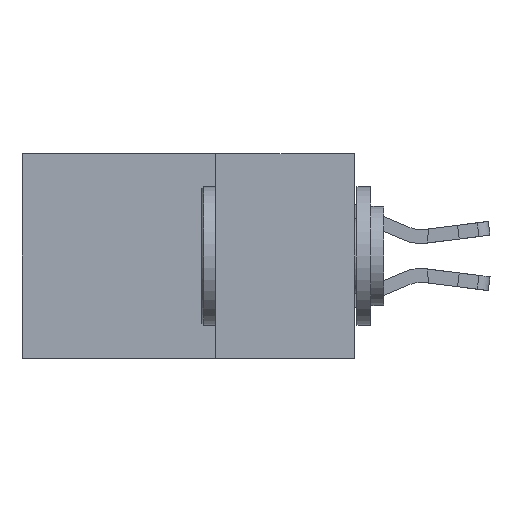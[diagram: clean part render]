
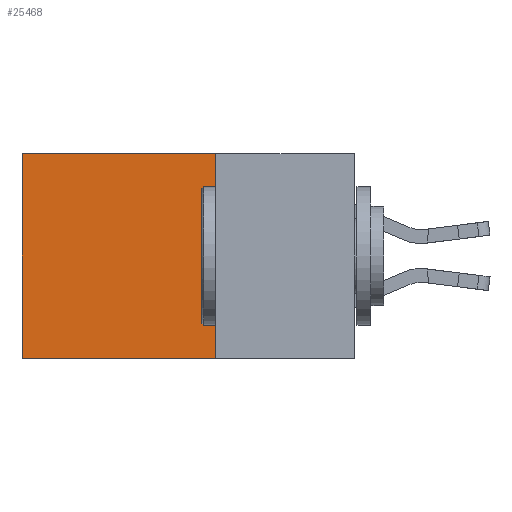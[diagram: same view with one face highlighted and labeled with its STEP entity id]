
A CAD part, left-side view. The second image highlights one B-rep face of the part: STEP entity #25468.
In plain terms, the highlighted planar face has unit normal (-1, 0, 0).
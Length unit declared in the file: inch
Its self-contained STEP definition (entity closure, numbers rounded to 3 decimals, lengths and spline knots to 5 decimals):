
#117 = CARTESIAN_POINT ( 'NONE',  ( 0.298, 0.25, 0. ) ) ;
#673 = EDGE_LOOP ( 'NONE', ( #4429, #25153, #6160, #6179 ) ) ;
#1301 = DIRECTION ( 'NONE',  ( 0., 0., -1. ) ) ;
#4429 = ORIENTED_EDGE ( 'NONE', *, *, #16541, .T. ) ;
#4519 = CARTESIAN_POINT ( 'NONE',  ( 0.298, 0.25, -0.37 ) ) ;
#5202 = LINE ( 'NONE', #8693, #21627 ) ;
#5887 = CARTESIAN_POINT ( 'NONE',  ( 0.298, 0.6, 0. ) ) ;
#6160 = ORIENTED_EDGE ( 'NONE', *, *, #19149, .F. ) ;
#6179 = ORIENTED_EDGE ( 'NONE', *, *, #23995, .T. ) ;
#6686 = VERTEX_POINT ( 'NONE', #5887 ) ;
#8188 = CARTESIAN_POINT ( 'NONE',  ( 0.298, 0.6, 0. ) ) ;
#8596 = FACE_OUTER_BOUND ( 'NONE', #673, .T. ) ;
#8693 = CARTESIAN_POINT ( 'NONE',  ( 0.298, 0.25, 0. ) ) ;
#9989 = CARTESIAN_POINT ( 'NONE',  ( 0.298, 0.25, 0. ) ) ;
#12301 = LINE ( 'NONE', #8188, #12620 ) ;
#12393 = DIRECTION ( 'NONE',  ( 1., 0., 0. ) ) ;
#12620 = VECTOR ( 'NONE', #23477, 39.37008 ) ;
#13023 = DIRECTION ( 'NONE',  ( 0., 0., -1. ) ) ;
#13510 = VERTEX_POINT ( 'NONE', #4519 ) ;
#13826 = CARTESIAN_POINT ( 'NONE',  ( 0.298, 0.25, -0.37 ) ) ;
#14691 = PLANE ( 'NONE',  #15583 ) ;
#15488 = DIRECTION ( 'NONE',  ( 0., 1., 0. ) ) ;
#15583 = AXIS2_PLACEMENT_3D ( 'NONE', #20888, #12393, #1301 ) ;
#16541 = EDGE_CURVE ( 'NONE', #6686, #23640, #12301, .T. ) ;
#17826 = EDGE_CURVE ( 'NONE', #13510, #23640, #19031, .T. ) ;
#18308 = DIRECTION ( 'NONE',  ( 0., 1., 0. ) ) ;
#18667 = VECTOR ( 'NONE', #13023, 39.37008 ) ;
#19031 = LINE ( 'NONE', #13826, #21098 ) ;
#19149 = EDGE_CURVE ( 'NONE', #22464, #13510, #24506, .T. ) ;
#20888 = CARTESIAN_POINT ( 'NONE',  ( 0.298, 0.25, 0. ) ) ;
#21098 = VECTOR ( 'NONE', #18308, 39.37008 ) ;
#21627 = VECTOR ( 'NONE', #15488, 39.37008 ) ;
#22464 = VERTEX_POINT ( 'NONE', #9989 ) ;
#23477 = DIRECTION ( 'NONE',  ( 0., 0., -1. ) ) ;
#23557 = CARTESIAN_POINT ( 'NONE',  ( 0.298, 0.6, -0.37 ) ) ;
#23640 = VERTEX_POINT ( 'NONE', #23557 ) ;
#23995 = EDGE_CURVE ( 'NONE', #22464, #6686, #5202, .T. ) ;
#24506 = LINE ( 'NONE', #117, #18667 ) ;
#25153 = ORIENTED_EDGE ( 'NONE', *, *, #17826, .F. ) ;
#25468 = ADVANCED_FACE ( 'NONE', ( #8596 ), #14691, .F. ) ;
